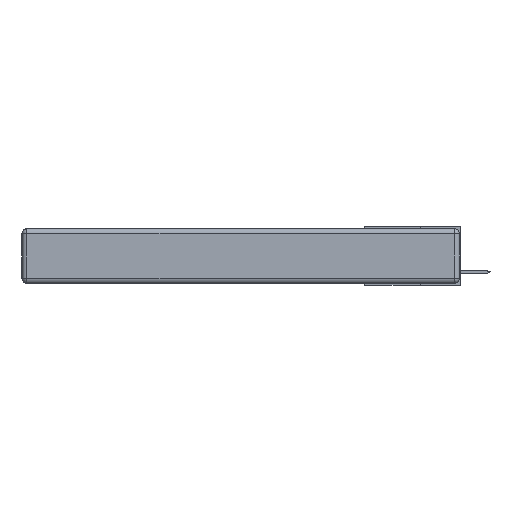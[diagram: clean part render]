
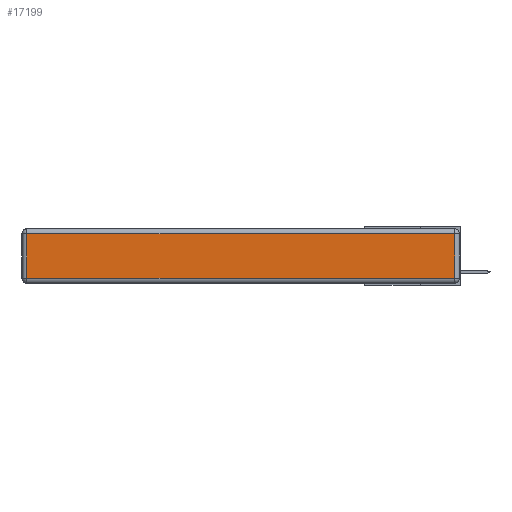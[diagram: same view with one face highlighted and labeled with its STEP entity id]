
A CAD part, left-side view. The second image highlights one B-rep face of the part: STEP entity #17199.
In plain terms, the highlighted planar face has unit normal (-1, 0, 0).
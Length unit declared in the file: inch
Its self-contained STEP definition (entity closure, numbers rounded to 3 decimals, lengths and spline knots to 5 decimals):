
#418 = VECTOR ( 'NONE', #14073, 39.37008 ) ;
#1146 = PLANE ( 'NONE',  #16853 ) ;
#1649 = DIRECTION ( 'NONE',  ( 0., 1., 0. ) ) ;
#1707 = CARTESIAN_POINT ( 'NONE',  ( 0., 0.03, -0.313 ) ) ;
#2021 = ORIENTED_EDGE ( 'NONE', *, *, #8023, .T. ) ;
#2448 = VERTEX_POINT ( 'NONE', #12056 ) ;
#3688 = VECTOR ( 'NONE', #1649, 39.37008 ) ;
#4010 = VERTEX_POINT ( 'NONE', #14972 ) ;
#4140 = ORIENTED_EDGE ( 'NONE', *, *, #11187, .T. ) ;
#4205 = DIRECTION ( 'NONE',  ( 0., 0., -1. ) ) ;
#4970 = CARTESIAN_POINT ( 'NONE',  ( 0., 0., -0.313 ) ) ;
#5301 = VECTOR ( 'NONE', #14971, 39.37008 ) ;
#5464 = EDGE_LOOP ( 'NONE', ( #10475, #4140, #12827, #2021 ) ) ;
#6766 = DIRECTION ( 'NONE',  ( -1., 0., 0. ) ) ;
#8023 = EDGE_CURVE ( 'NONE', #2448, #4010, #14389, .T. ) ;
#8859 = FACE_OUTER_BOUND ( 'NONE', #5464, .T. ) ;
#9747 = CARTESIAN_POINT ( 'NONE',  ( 0., 0.03, -0.343 ) ) ;
#10109 = VECTOR ( 'NONE', #4205, 39.37008 ) ;
#10475 = ORIENTED_EDGE ( 'NONE', *, *, #15700, .T. ) ;
#11187 = EDGE_CURVE ( 'NONE', #17435, #11213, #13106, .T. ) ;
#11213 = VERTEX_POINT ( 'NONE', #17786 ) ;
#11374 = CARTESIAN_POINT ( 'NONE',  ( 0., 2.72, -0.343 ) ) ;
#12056 = CARTESIAN_POINT ( 'NONE',  ( 0., 2.72, -0.03 ) ) ;
#12827 = ORIENTED_EDGE ( 'NONE', *, *, #15452, .T. ) ;
#13106 = LINE ( 'NONE', #9747, #418 ) ;
#13421 = LINE ( 'NONE', #17709, #3688 ) ;
#14021 = DIRECTION ( 'NONE',  ( 0., 0., 1. ) ) ;
#14073 = DIRECTION ( 'NONE',  ( 0., 0., 1. ) ) ;
#14389 = LINE ( 'NONE', #11374, #10109 ) ;
#14971 = DIRECTION ( 'NONE',  ( 0., -1., 0. ) ) ;
#14972 = CARTESIAN_POINT ( 'NONE',  ( 0., 2.72, -0.313 ) ) ;
#15237 = LINE ( 'NONE', #4970, #5301 ) ;
#15452 = EDGE_CURVE ( 'NONE', #11213, #2448, #13421, .T. ) ;
#15700 = EDGE_CURVE ( 'NONE', #4010, #17435, #15237, .T. ) ;
#16853 = AXIS2_PLACEMENT_3D ( 'NONE', #16978, #6766, #14021 ) ;
#16978 = CARTESIAN_POINT ( 'NONE',  ( 0., 0., -0.343 ) ) ;
#17199 = ADVANCED_FACE ( 'NONE', ( #8859 ), #1146, .T. ) ;
#17435 = VERTEX_POINT ( 'NONE', #1707 ) ;
#17709 = CARTESIAN_POINT ( 'NONE',  ( 0., 2.75, -0.03 ) ) ;
#17786 = CARTESIAN_POINT ( 'NONE',  ( 0., 0.03, -0.03 ) ) ;
